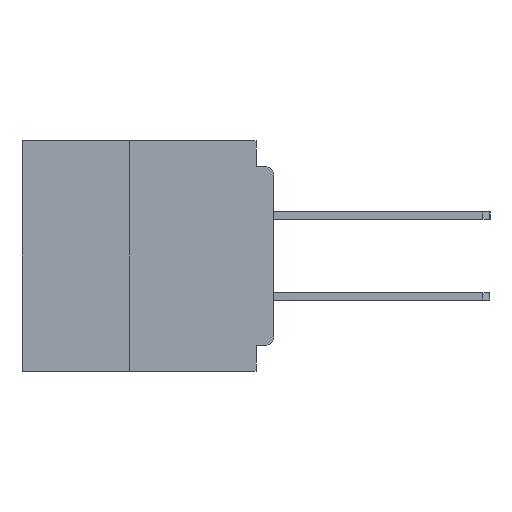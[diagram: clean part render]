
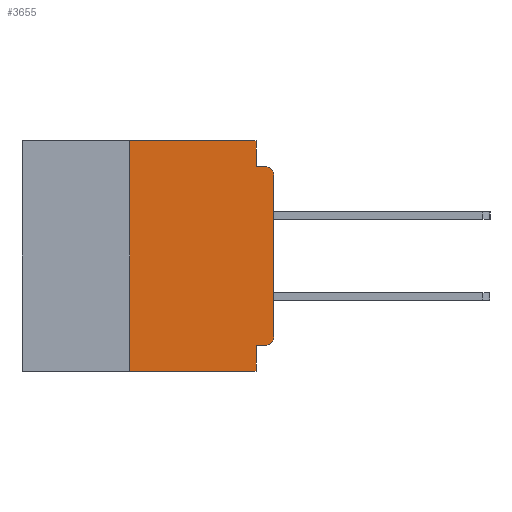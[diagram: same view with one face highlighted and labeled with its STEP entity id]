
A CAD part, left-side view. The second image highlights one B-rep face of the part: STEP entity #3655.
In plain terms, the highlighted planar face has unit normal (-1, 0, 0).
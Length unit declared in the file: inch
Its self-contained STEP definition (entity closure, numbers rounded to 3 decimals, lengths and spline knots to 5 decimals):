
#222 = CARTESIAN_POINT ( 'NONE',  ( 0., 0.015, -0.34 ) ) ;
#826 = ORIENTED_EDGE ( 'NONE', *, *, #56069, .T. ) ;
#1389 = ORIENTED_EDGE ( 'NONE', *, *, #58853, .F. ) ;
#3008 = CARTESIAN_POINT ( 'NONE',  ( 0., 0.437, 0. ) ) ;
#3148 = LINE ( 'NONE', #19340, #52598 ) ;
#3655 = ADVANCED_FACE ( 'NONE', ( #34256 ), #15338, .F. ) ;
#3972 = VERTEX_POINT ( 'NONE', #5627 ) ;
#4691 = ORIENTED_EDGE ( 'NONE', *, *, #58303, .F. ) ;
#4749 = VERTEX_POINT ( 'NONE', #46954 ) ;
#4996 = DIRECTION ( 'NONE',  ( 0., 0., -1. ) ) ;
#5524 = VERTEX_POINT ( 'NONE', #29562 ) ;
#5542 = DIRECTION ( 'NONE',  ( 0., 0., -1. ) ) ;
#5627 = CARTESIAN_POINT ( 'NONE',  ( 0., 0.031, -0.355 ) ) ;
#6430 = VECTOR ( 'NONE', #43293, 39.37008 ) ;
#6971 = ORIENTED_EDGE ( 'NONE', *, *, #34537, .F. ) ;
#9161 = VERTEX_POINT ( 'NONE', #31385 ) ;
#11436 = EDGE_CURVE ( 'NONE', #4749, #53204, #27220, .T. ) ;
#12152 = DIRECTION ( 'NONE',  ( 0., 0., 1. ) ) ;
#13733 = EDGE_CURVE ( 'NONE', #16794, #9161, #32873, .T. ) ;
#14207 = VECTOR ( 'NONE', #30774, 39.37008 ) ;
#14591 = CARTESIAN_POINT ( 'NONE',  ( 0., 0.015, -0.06 ) ) ;
#14640 = VERTEX_POINT ( 'NONE', #28705 ) ;
#14996 = CARTESIAN_POINT ( 'NONE',  ( 0., 0.031, -0.4 ) ) ;
#15272 = DIRECTION ( 'NONE',  ( 0., 0., -1. ) ) ;
#15338 = PLANE ( 'NONE',  #55429 ) ;
#15490 = CARTESIAN_POINT ( 'NONE',  ( 0., 0.437, 0. ) ) ;
#15712 = DIRECTION ( 'NONE',  ( 1., 0., 0. ) ) ;
#15804 = LINE ( 'NONE', #55010, #41293 ) ;
#16794 = VERTEX_POINT ( 'NONE', #51533 ) ;
#17849 = AXIS2_PLACEMENT_3D ( 'NONE', #14591, #48043, #19430 ) ;
#18676 = CARTESIAN_POINT ( 'NONE',  ( 0., 0.015, -0.045 ) ) ;
#18797 = ORIENTED_EDGE ( 'NONE', *, *, #59200, .F. ) ;
#19340 = CARTESIAN_POINT ( 'NONE',  ( 0., 0.031, 0. ) ) ;
#19430 = DIRECTION ( 'NONE',  ( 0., 0., -1. ) ) ;
#24190 = CARTESIAN_POINT ( 'NONE',  ( 0., 0.031, -0.4 ) ) ;
#25971 = CARTESIAN_POINT ( 'NONE',  ( 0., 0., -0.355 ) ) ;
#26352 = DIRECTION ( 'NONE',  ( 0., -1., 0. ) ) ;
#26384 = LINE ( 'NONE', #50245, #48817 ) ;
#27206 = ORIENTED_EDGE ( 'NONE', *, *, #58596, .T. ) ;
#27220 = CIRCLE ( 'NONE', #38418, 0.015 ) ;
#27295 = VECTOR ( 'NONE', #5542, 39.37008 ) ;
#28467 = LINE ( 'NONE', #25971, #14207 ) ;
#28705 = CARTESIAN_POINT ( 'NONE',  ( 0., 0., -0.06 ) ) ;
#28952 = CIRCLE ( 'NONE', #17849, 0.015 ) ;
#29562 = CARTESIAN_POINT ( 'NONE',  ( 0., 0.031, -0.045 ) ) ;
#30186 = EDGE_CURVE ( 'NONE', #49272, #53278, #44654, .T. ) ;
#30774 = DIRECTION ( 'NONE',  ( 0., 1., 0. ) ) ;
#31385 = CARTESIAN_POINT ( 'NONE',  ( 0., 0.031, 0. ) ) ;
#32873 = LINE ( 'NONE', #3008, #56816 ) ;
#33718 = DIRECTION ( 'NONE',  ( -1., 0., 0. ) ) ;
#34245 = VERTEX_POINT ( 'NONE', #18676 ) ;
#34256 = FACE_OUTER_BOUND ( 'NONE', #50458, .T. ) ;
#34537 = EDGE_CURVE ( 'NONE', #4749, #3972, #28467, .T. ) ;
#38355 = ORIENTED_EDGE ( 'NONE', *, *, #13733, .F. ) ;
#38418 = AXIS2_PLACEMENT_3D ( 'NONE', #222, #33718, #4996 ) ;
#38485 = CARTESIAN_POINT ( 'NONE',  ( 0., 0.437, -0.4 ) ) ;
#41293 = VECTOR ( 'NONE', #26352, 39.37008 ) ;
#43293 = DIRECTION ( 'NONE',  ( 0., -1., 0. ) ) ;
#43859 = ORIENTED_EDGE ( 'NONE', *, *, #61452, .F. ) ;
#44654 = LINE ( 'NONE', #38485, #6430 ) ;
#46512 = VECTOR ( 'NONE', #52313, 39.37008 ) ;
#46954 = CARTESIAN_POINT ( 'NONE',  ( 0., 0.015, -0.355 ) ) ;
#48043 = DIRECTION ( 'NONE',  ( -1., 0., 0. ) ) ;
#48177 = DIRECTION ( 'NONE',  ( 0., 0., -1. ) ) ;
#48817 = VECTOR ( 'NONE', #12152, 39.37008 ) ;
#49272 = VERTEX_POINT ( 'NONE', #56766 ) ;
#50245 = CARTESIAN_POINT ( 'NONE',  ( 0., 0., 0. ) ) ;
#50458 = EDGE_LOOP ( 'NONE', ( #27206, #826, #18797, #4691, #38355, #1389, #57226, #43859, #6971, #60206 ) ) ;
#51533 = CARTESIAN_POINT ( 'NONE',  ( 0., 0.25, 0. ) ) ;
#52313 = DIRECTION ( 'NONE',  ( 0., 0., 1. ) ) ;
#52598 = VECTOR ( 'NONE', #48177, 39.37008 ) ;
#52741 = LINE ( 'NONE', #14996, #27295 ) ;
#53204 = VERTEX_POINT ( 'NONE', #61842 ) ;
#53278 = VERTEX_POINT ( 'NONE', #24190 ) ;
#55010 = CARTESIAN_POINT ( 'NONE',  ( 0., 0., -0.045 ) ) ;
#55429 = AXIS2_PLACEMENT_3D ( 'NONE', #15490, #15712, #15272 ) ;
#56069 = EDGE_CURVE ( 'NONE', #14640, #34245, #28952, .T. ) ;
#56766 = CARTESIAN_POINT ( 'NONE',  ( 0., 0.25, -0.4 ) ) ;
#56816 = VECTOR ( 'NONE', #60380, 39.37008 ) ;
#57140 = CARTESIAN_POINT ( 'NONE',  ( 0., 0.25, -0.4 ) ) ;
#57226 = ORIENTED_EDGE ( 'NONE', *, *, #30186, .T. ) ;
#58303 = EDGE_CURVE ( 'NONE', #9161, #5524, #3148, .T. ) ;
#58596 = EDGE_CURVE ( 'NONE', #53204, #14640, #26384, .T. ) ;
#58853 = EDGE_CURVE ( 'NONE', #49272, #16794, #59285, .T. ) ;
#59200 = EDGE_CURVE ( 'NONE', #5524, #34245, #15804, .T. ) ;
#59285 = LINE ( 'NONE', #57140, #46512 ) ;
#60206 = ORIENTED_EDGE ( 'NONE', *, *, #11436, .T. ) ;
#60380 = DIRECTION ( 'NONE',  ( 0., -1., 0. ) ) ;
#61452 = EDGE_CURVE ( 'NONE', #3972, #53278, #52741, .T. ) ;
#61842 = CARTESIAN_POINT ( 'NONE',  ( 0., 0., -0.34 ) ) ;
